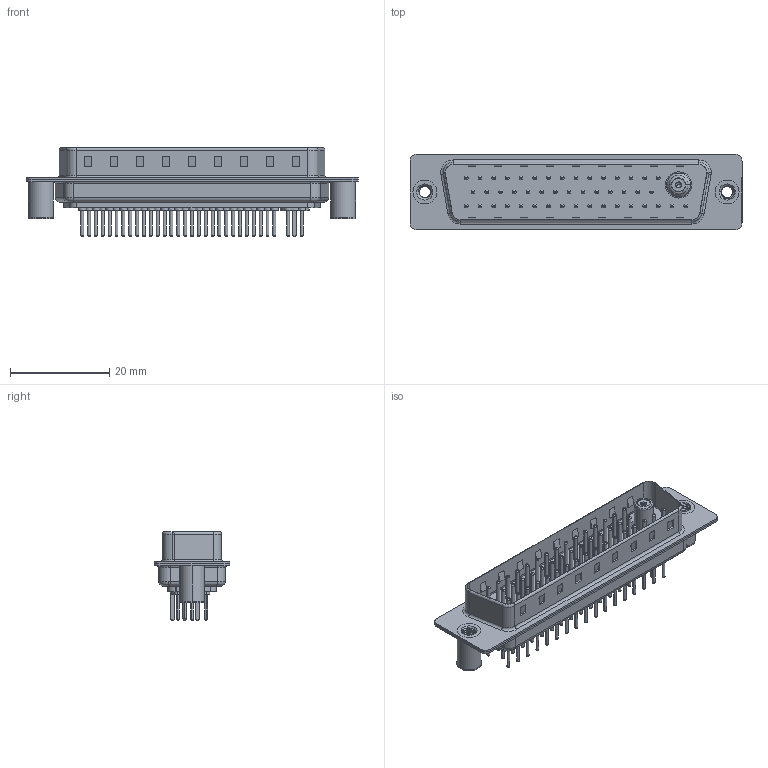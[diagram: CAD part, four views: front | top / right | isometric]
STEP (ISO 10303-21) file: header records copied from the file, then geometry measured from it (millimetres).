
FILE_DESCRIPTION (( 'STEP AP203' ), '1' );
FILE_NAME ('627-47W1224-7NB.STEP', '2019-06-20T16:15:11', ( '' ), ( '' ), 'SwSTEP 2.0', 'SolidWorks 2016', '' );
FILE_SCHEMA (( 'CONFIG_CONTROL_DESIGN' ));
Length unit declared in the file: millimetre
Products named in the file (15): Co-Ax Jack_Straight PC Tail; 627Combo Housing_47W1; 627Combo Threaded Board Spacer_B; 627Combo Contact Row 2_24; 627Combo Shell Front_50 Contacts; Co-Ax Jack Assy_St; 627Combo Contact Row 1_24; 627Combo Contact Row 3_24; 627Combo Shell Rear_50 Contacts; Socket_Str; 627Combo Threaded Board Spacer_3; Insulator Socket; Locking Collar; 627-47W1224-7NB; Insulator Socket 2
Assembly tree (57 placements, depth 3):
  627-47W1224-7NB
    627Combo Housing_47W1
    627Combo Shell Rear_50 Contacts
    627Combo Shell Front_50 Contacts
    627Combo Threaded Board Spacer_B
    Co-Ax Jack Assy_St
      Co-Ax Jack_Straight PC Tail
      Insulator Socket
      Insulator Socket 2
      Locking Collar
      Socket_Str
    627Combo Threaded Board Spacer_3
    627Combo Contact Row 1_24  x15
    627Combo Contact Row 2_24  x14
    627Combo Contact Row 3_24  x17
Bounding box: 67 x 15.3 x 17.9 mm (x, y, z)
Volume: 4672.4 mm3; surface area: 11436.1 mm2
Topology: 56 solids, 56 shells, 2263 faces, 4805 edges, 2903 vertices
Faces by surface type: cylinder 860, torus 794, plane 572, cone 27, bspline 8, sphere 2
Entity records: 36200 total; most frequent: CARTESIAN_POINT 8882, DIRECTION 5562, ORIENTED_EDGE 4782, EDGE_CURVE 2391, AXIS2_PLACEMENT_3D 2232, VERTEX_POINT 1527, EDGE_LOOP 1294, CIRCLE 1163
